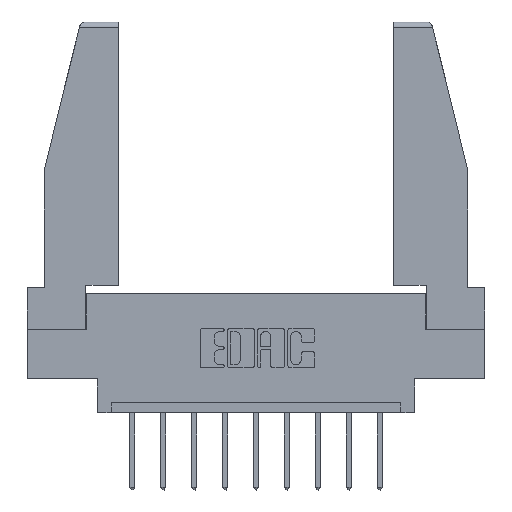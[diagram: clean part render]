
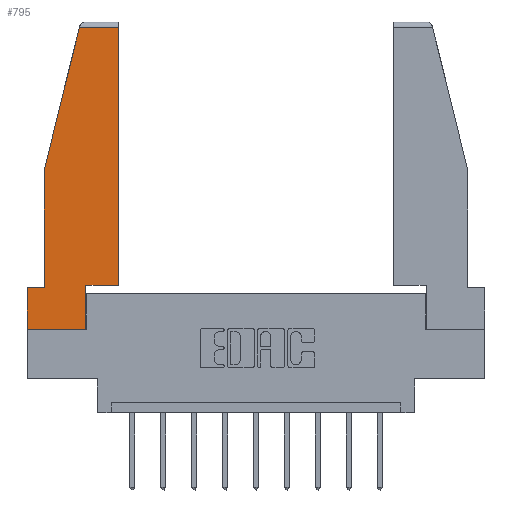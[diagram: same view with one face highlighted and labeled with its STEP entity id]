
A CAD part, top view. The second image highlights one B-rep face of the part: STEP entity #795.
In plain terms, the highlighted planar face has unit normal (0, 0, 1).
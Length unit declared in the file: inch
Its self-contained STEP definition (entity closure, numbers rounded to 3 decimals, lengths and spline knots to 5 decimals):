
#14 = LINE ( 'NONE', #5150, #1825 ) ;
#222 = DIRECTION ( 'NONE',  ( 1., 0., 0. ) ) ;
#242 = EDGE_CURVE ( 'NONE', #8009, #7983, #4865, .T. ) ;
#559 = LINE ( 'NONE', #13305, #10698 ) ;
#606 = VERTEX_POINT ( 'NONE', #10760 ) ;
#738 = CARTESIAN_POINT ( 'NONE',  ( 0.297, 0.223, 0. ) ) ;
#795 = ADVANCED_FACE ( 'NONE', ( #12364 ), #3246, .T. ) ;
#1145 = DIRECTION ( 'NONE',  ( 1., 0., 0. ) ) ;
#1341 = LINE ( 'NONE', #4133, #9815 ) ;
#1404 = ORIENTED_EDGE ( 'NONE', *, *, #12941, .T. ) ;
#1628 = CARTESIAN_POINT ( 'NONE',  ( 0., 0.21, 0. ) ) ;
#1710 = CARTESIAN_POINT ( 'NONE',  ( 0.2636, 1.52, 0. ) ) ;
#1825 = VECTOR ( 'NONE', #7202, 39.37008 ) ;
#1929 = DIRECTION ( 'NONE',  ( -0.239, -0.971, 0. ) ) ;
#2136 = VECTOR ( 'NONE', #3697, 39.37008 ) ;
#2317 = VERTEX_POINT ( 'NONE', #4438 ) ;
#2969 = VECTOR ( 'NONE', #10597, 39.37008 ) ;
#3013 = VECTOR ( 'NONE', #11675, 39.37008 ) ;
#3246 = PLANE ( 'NONE',  #10211 ) ;
#3438 = VERTEX_POINT ( 'NONE', #4374 ) ;
#3505 = ORIENTED_EDGE ( 'NONE', *, *, #3605, .T. ) ;
#3518 = EDGE_CURVE ( 'NONE', #4911, #12116, #14, .T. ) ;
#3605 = EDGE_CURVE ( 'NONE', #6293, #4911, #1341, .T. ) ;
#3697 = DIRECTION ( 'NONE',  ( -1., 0., 0. ) ) ;
#4053 = VERTEX_POINT ( 'NONE', #9775 ) ;
#4078 = CARTESIAN_POINT ( 'NONE',  ( 0., 1.52, 0. ) ) ;
#4133 = CARTESIAN_POINT ( 'NONE',  ( 0.271, 1.55, 0. ) ) ;
#4137 = LINE ( 'NONE', #5430, #13453 ) ;
#4279 = ORIENTED_EDGE ( 'NONE', *, *, #11526, .T. ) ;
#4374 = CARTESIAN_POINT ( 'NONE',  ( 0.461, 1.52, 0. ) ) ;
#4438 = CARTESIAN_POINT ( 'NONE',  ( 0., 0.21, 0. ) ) ;
#4772 = LINE ( 'NONE', #5323, #2969 ) ;
#4778 = EDGE_LOOP ( 'NONE', ( #11244, #10422, #3505, #12079, #11371, #1404, #10247, #4279, #13247 ) ) ;
#4865 = LINE ( 'NONE', #10559, #10568 ) ;
#4911 = VERTEX_POINT ( 'NONE', #13312 ) ;
#5150 = CARTESIAN_POINT ( 'NONE',  ( 0.086, 0.8, 0. ) ) ;
#5323 = CARTESIAN_POINT ( 'NONE',  ( 0., 0.21, 0. ) ) ;
#5430 = CARTESIAN_POINT ( 'NONE',  ( 0.461, 0.223, 0. ) ) ;
#5894 = CARTESIAN_POINT ( 'NONE',  ( 0.086, 0.21, 0. ) ) ;
#6293 = VERTEX_POINT ( 'NONE', #1710 ) ;
#6468 = EDGE_CURVE ( 'NONE', #4053, #606, #559, .T. ) ;
#7081 = DIRECTION ( 'NONE',  ( 1., 0., 0. ) ) ;
#7202 = DIRECTION ( 'NONE',  ( 0., -1., 0. ) ) ;
#7983 = VERTEX_POINT ( 'NONE', #9728 ) ;
#8009 = VERTEX_POINT ( 'NONE', #738 ) ;
#8172 = EDGE_CURVE ( 'NONE', #3438, #6293, #10657, .T. ) ;
#8597 = DIRECTION ( 'NONE',  ( 0., 0., 1. ) ) ;
#9088 = EDGE_CURVE ( 'NONE', #12116, #2317, #13261, .T. ) ;
#9175 = VECTOR ( 'NONE', #11396, 39.37008 ) ;
#9582 = DIRECTION ( 'NONE',  ( 0., 1., 0. ) ) ;
#9728 = CARTESIAN_POINT ( 'NONE',  ( 0.461, 0.223, 0. ) ) ;
#9775 = CARTESIAN_POINT ( 'NONE',  ( 0., 0., 0. ) ) ;
#9815 = VECTOR ( 'NONE', #1929, 39.37008 ) ;
#10211 = AXIS2_PLACEMENT_3D ( 'NONE', #12616, #8597, #1145 ) ;
#10247 = ORIENTED_EDGE ( 'NONE', *, *, #6468, .T. ) ;
#10422 = ORIENTED_EDGE ( 'NONE', *, *, #8172, .T. ) ;
#10559 = CARTESIAN_POINT ( 'NONE',  ( 0.297, 0.223, 0. ) ) ;
#10568 = VECTOR ( 'NONE', #222, 39.37008 ) ;
#10597 = DIRECTION ( 'NONE',  ( 0., -1., 0. ) ) ;
#10657 = LINE ( 'NONE', #4078, #9175 ) ;
#10698 = VECTOR ( 'NONE', #7081, 39.37008 ) ;
#10753 = CARTESIAN_POINT ( 'NONE',  ( 0.297, 0., 0. ) ) ;
#10760 = CARTESIAN_POINT ( 'NONE',  ( 0.297, 0., 0. ) ) ;
#11244 = ORIENTED_EDGE ( 'NONE', *, *, #12445, .T. ) ;
#11371 = ORIENTED_EDGE ( 'NONE', *, *, #9088, .T. ) ;
#11396 = DIRECTION ( 'NONE',  ( -1., 0., 0. ) ) ;
#11526 = EDGE_CURVE ( 'NONE', #606, #8009, #11689, .T. ) ;
#11675 = DIRECTION ( 'NONE',  ( 0., 1., 0. ) ) ;
#11689 = LINE ( 'NONE', #10753, #3013 ) ;
#12079 = ORIENTED_EDGE ( 'NONE', *, *, #3518, .T. ) ;
#12116 = VERTEX_POINT ( 'NONE', #5894 ) ;
#12364 = FACE_OUTER_BOUND ( 'NONE', #4778, .T. ) ;
#12445 = EDGE_CURVE ( 'NONE', #7983, #3438, #4137, .T. ) ;
#12616 = CARTESIAN_POINT ( 'NONE',  ( 0., 0., 0. ) ) ;
#12941 = EDGE_CURVE ( 'NONE', #2317, #4053, #4772, .T. ) ;
#13247 = ORIENTED_EDGE ( 'NONE', *, *, #242, .T. ) ;
#13261 = LINE ( 'NONE', #1628, #2136 ) ;
#13305 = CARTESIAN_POINT ( 'NONE',  ( 0., 0., 0. ) ) ;
#13312 = CARTESIAN_POINT ( 'NONE',  ( 0.086, 0.8, 0. ) ) ;
#13453 = VECTOR ( 'NONE', #9582, 39.37008 ) ;
